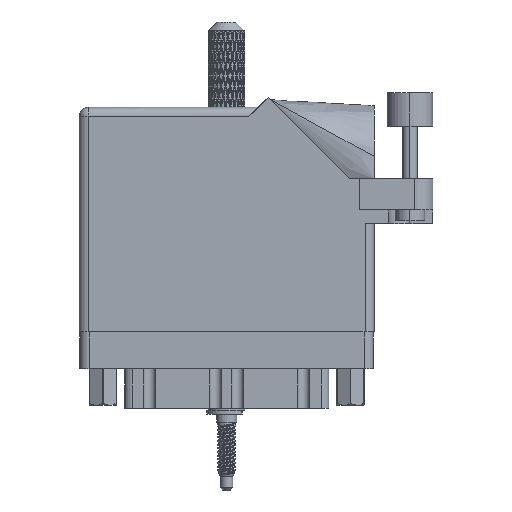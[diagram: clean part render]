
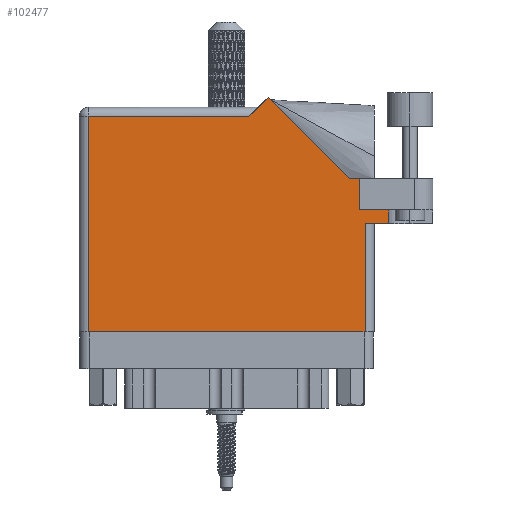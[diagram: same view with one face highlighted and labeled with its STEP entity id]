
A CAD part, front view. The second image highlights one B-rep face of the part: STEP entity #102477.
In plain terms, the highlighted face is planar.
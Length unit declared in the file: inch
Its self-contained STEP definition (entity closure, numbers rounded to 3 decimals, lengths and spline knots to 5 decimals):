
#1218 = LINE ( 'NONE', #45484, #42924 ) ;
#2314 = DIRECTION ( 'NONE',  ( -1., 0., 0. ) ) ;
#2880 = PLANE ( 'NONE',  #75876 ) ;
#3555 = ORIENTED_EDGE ( 'NONE', *, *, #82284, .F. ) ;
#3982 = VERTEX_POINT ( 'NONE', #34439 ) ;
#5011 = CARTESIAN_POINT ( 'NONE',  ( 1.91, 1.044, 0. ) ) ;
#6336 = CARTESIAN_POINT ( 'NONE',  ( 0.062, 0., 0. ) ) ;
#6440 = CARTESIAN_POINT ( 'NONE',  ( 1.91, 0.831, 0. ) ) ;
#6756 = VERTEX_POINT ( 'NONE', #80588 ) ;
#6806 = CARTESIAN_POINT ( 'NONE',  ( 1.948, 0.737, 0. ) ) ;
#8102 = LINE ( 'NONE', #43195, #57557 ) ;
#8740 = CARTESIAN_POINT ( 'NONE',  ( 1.91, 0.831, 0. ) ) ;
#8925 = VERTEX_POINT ( 'NONE', #10444 ) ;
#9761 = VECTOR ( 'NONE', #78255, 39.37008 ) ;
#10444 = CARTESIAN_POINT ( 'NONE',  ( 2.1115, 0.737, 0. ) ) ;
#10667 = ORIENTED_EDGE ( 'NONE', *, *, #104628, .T. ) ;
#11528 = DIRECTION ( 'NONE',  ( 0., 0., -1. ) ) ;
#14626 = VERTEX_POINT ( 'NONE', #46442 ) ;
#14635 = EDGE_CURVE ( 'NONE', #3982, #97032, #81507, .T. ) ;
#15994 = DIRECTION ( 'NONE',  ( -0.707, 0.707, 0. ) ) ;
#18863 = VECTOR ( 'NONE', #63997, 39.37008 ) ;
#19146 = EDGE_LOOP ( 'NONE', ( #107763, #40562, #23110, #48134, #3555, #41858, #44594, #10667, #49244, #63580, #60664 ) ) ;
#19182 = CARTESIAN_POINT ( 'NONE',  ( 2.01, 0.737, 0. ) ) ;
#22646 = EDGE_CURVE ( 'NONE', #51613, #30444, #102457, .T. ) ;
#23110 = ORIENTED_EDGE ( 'NONE', *, *, #43490, .T. ) ;
#24598 = LINE ( 'NONE', #59662, #50354 ) ;
#24637 = LINE ( 'NONE', #6806, #95417 ) ;
#27089 = CARTESIAN_POINT ( 'NONE',  ( 0., 0., 0. ) ) ;
#28471 = VECTOR ( 'NONE', #79824, 39.37008 ) ;
#30444 = VERTEX_POINT ( 'NONE', #5011 ) ;
#34223 = DIRECTION ( 'NONE',  ( 0., -1., 0. ) ) ;
#34439 = CARTESIAN_POINT ( 'NONE',  ( 1.155, 1.468, 0. ) ) ;
#34610 = FACE_OUTER_BOUND ( 'NONE', #19146, .T. ) ;
#36325 = DIRECTION ( 'NONE',  ( -0.707, -0.707, 0. ) ) ;
#38298 = DIRECTION ( 'NONE',  ( -1., 0., 0. ) ) ;
#40562 = ORIENTED_EDGE ( 'NONE', *, *, #100693, .T. ) ;
#41446 = VERTEX_POINT ( 'NONE', #58984 ) ;
#41858 = ORIENTED_EDGE ( 'NONE', *, *, #22646, .T. ) ;
#42924 = VECTOR ( 'NONE', #36325, 39.37008 ) ;
#43195 = CARTESIAN_POINT ( 'NONE',  ( 2.1115, 1.16177, 0. ) ) ;
#43490 = EDGE_CURVE ( 'NONE', #6756, #8925, #70912, .T. ) ;
#44594 = ORIENTED_EDGE ( 'NONE', *, *, #48110, .T. ) ;
#45476 = CARTESIAN_POINT ( 'NONE',  ( 1.948, 0., 0. ) ) ;
#45484 = CARTESIAN_POINT ( 'NONE',  ( 1.217, 1.53, 0. ) ) ;
#46442 = CARTESIAN_POINT ( 'NONE',  ( 2.1115, 0.831, 0. ) ) ;
#48110 = EDGE_CURVE ( 'NONE', #30444, #41446, #55484, .T. ) ;
#48134 = ORIENTED_EDGE ( 'NONE', *, *, #49542, .F. ) ;
#49244 = ORIENTED_EDGE ( 'NONE', *, *, #50150, .T. ) ;
#49542 = EDGE_CURVE ( 'NONE', #14626, #8925, #8102, .T. ) ;
#49602 = VECTOR ( 'NONE', #34223, 39.37008 ) ;
#50150 = EDGE_CURVE ( 'NONE', #60533, #3982, #1218, .T. ) ;
#50354 = VECTOR ( 'NONE', #15994, 39.37008 ) ;
#51613 = VERTEX_POINT ( 'NONE', #88871 ) ;
#55202 = CARTESIAN_POINT ( 'NONE',  ( 0., 1.53, 0. ) ) ;
#55369 = EDGE_CURVE ( 'NONE', #78507, #55566, #85151, .T. ) ;
#55484 = LINE ( 'NONE', #64697, #105424 ) ;
#55566 = VERTEX_POINT ( 'NONE', #45476 ) ;
#57557 = VECTOR ( 'NONE', #104707, 39.37008 ) ;
#58984 = CARTESIAN_POINT ( 'NONE',  ( 1.84442, 1.044, 0. ) ) ;
#59662 = CARTESIAN_POINT ( 'NONE',  ( 1.84442, 1.044, 0. ) ) ;
#60533 = VERTEX_POINT ( 'NONE', #66287 ) ;
#60664 = ORIENTED_EDGE ( 'NONE', *, *, #82977, .T. ) ;
#61630 = DIRECTION ( 'NONE',  ( 1., 0., 0. ) ) ;
#63580 = ORIENTED_EDGE ( 'NONE', *, *, #14635, .T. ) ;
#63997 = DIRECTION ( 'NONE',  ( 1., 0., 0. ) ) ;
#64697 = CARTESIAN_POINT ( 'NONE',  ( 2.41, 1.044, 0. ) ) ;
#66287 = CARTESIAN_POINT ( 'NONE',  ( 1.28771, 1.60071, 0. ) ) ;
#69128 = CARTESIAN_POINT ( 'NONE',  ( 0.062, 1.468, 0. ) ) ;
#69691 = LINE ( 'NONE', #8740, #102782 ) ;
#70912 = LINE ( 'NONE', #19182, #18863 ) ;
#72886 = CARTESIAN_POINT ( 'NONE',  ( 0., 1.468, 0. ) ) ;
#75876 = AXIS2_PLACEMENT_3D ( 'NONE', #55202, #11528, #2314 ) ;
#76324 = LINE ( 'NONE', #111415, #49602 ) ;
#78255 = DIRECTION ( 'NONE',  ( 1., 0., 0. ) ) ;
#78507 = VERTEX_POINT ( 'NONE', #6336 ) ;
#79824 = DIRECTION ( 'NONE',  ( -1., 0., 0. ) ) ;
#80588 = CARTESIAN_POINT ( 'NONE',  ( 1.948, 0.737, 0. ) ) ;
#81507 = LINE ( 'NONE', #72886, #28471 ) ;
#82284 = EDGE_CURVE ( 'NONE', #51613, #14626, #69691, .T. ) ;
#82977 = EDGE_CURVE ( 'NONE', #97032, #78507, #76324, .T. ) ;
#85151 = LINE ( 'NONE', #27089, #9761 ) ;
#85185 = DIRECTION ( 'NONE',  ( 0., 1., 0. ) ) ;
#88871 = CARTESIAN_POINT ( 'NONE',  ( 1.91, 0.831, 0. ) ) ;
#94755 = DIRECTION ( 'NONE',  ( 0., 1., 0. ) ) ;
#95417 = VECTOR ( 'NONE', #94755, 39.37008 ) ;
#97032 = VERTEX_POINT ( 'NONE', #69128 ) ;
#100693 = EDGE_CURVE ( 'NONE', #55566, #6756, #24637, .T. ) ;
#102457 = LINE ( 'NONE', #6440, #105399 ) ;
#102477 = ADVANCED_FACE ( 'NONE', ( #34610 ), #2880, .F. ) ;
#102782 = VECTOR ( 'NONE', #61630, 39.37008 ) ;
#104628 = EDGE_CURVE ( 'NONE', #41446, #60533, #24598, .T. ) ;
#104707 = DIRECTION ( 'NONE',  ( 0., -1., 0. ) ) ;
#105399 = VECTOR ( 'NONE', #85185, 39.37008 ) ;
#105424 = VECTOR ( 'NONE', #38298, 39.37008 ) ;
#107763 = ORIENTED_EDGE ( 'NONE', *, *, #55369, .T. ) ;
#111415 = CARTESIAN_POINT ( 'NONE',  ( 0.062, 0., 0. ) ) ;
